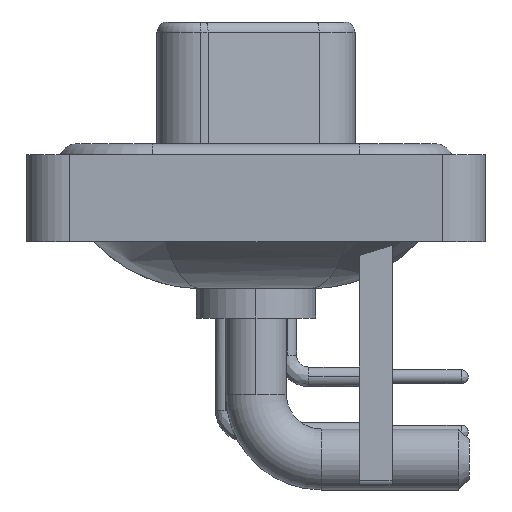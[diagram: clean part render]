
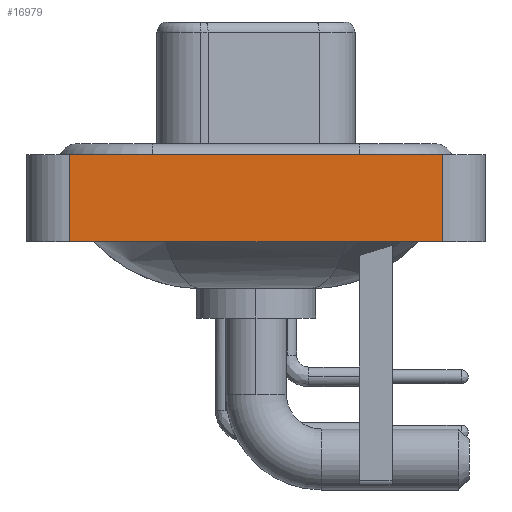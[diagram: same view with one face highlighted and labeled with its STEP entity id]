
A CAD part, left-side view. The second image highlights one B-rep face of the part: STEP entity #16979.
In plain terms, the highlighted planar face has unit normal (-1, 0, 0).
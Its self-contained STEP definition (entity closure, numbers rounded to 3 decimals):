
#830 = PLANE ( 'NONE',  #2655 ) ;
#1372 = LINE ( 'NONE', #16471, #21326 ) ;
#1569 = CARTESIAN_POINT ( 'NONE',  ( -7.3, 8.55, -3.6 ) ) ;
#2655 = AXIS2_PLACEMENT_3D ( 'NONE', #10291, #4549, #4817 ) ;
#2939 = CARTESIAN_POINT ( 'NONE',  ( -7.3, -8.55, 0.4 ) ) ;
#4549 = DIRECTION ( 'NONE',  ( -1., 0., 0. ) ) ;
#4817 = DIRECTION ( 'NONE',  ( 0., 0., 1. ) ) ;
#4832 = ORIENTED_EDGE ( 'NONE', *, *, #13783, .F. ) ;
#4885 = CARTESIAN_POINT ( 'NONE',  ( -7.3, 8.55, -3.6 ) ) ;
#4992 = DIRECTION ( 'NONE',  ( 0., -1., 0. ) ) ;
#5637 = VECTOR ( 'NONE', #4992, 1000. ) ;
#6269 = ORIENTED_EDGE ( 'NONE', *, *, #20563, .T. ) ;
#6390 = VERTEX_POINT ( 'NONE', #25256 ) ;
#6558 = LINE ( 'NONE', #20486, #23531 ) ;
#8976 = DIRECTION ( 'NONE',  ( 0., 0., 1. ) ) ;
#9183 = DIRECTION ( 'NONE',  ( 0., 0., 1. ) ) ;
#9903 = VERTEX_POINT ( 'NONE', #14585 ) ;
#10291 = CARTESIAN_POINT ( 'NONE',  ( -7.3, -8.55, -3.6 ) ) ;
#12181 = DIRECTION ( 'NONE',  ( 0., -1., 0. ) ) ;
#13783 = EDGE_CURVE ( 'NONE', #9903, #20395, #18400, .T. ) ;
#14347 = ORIENTED_EDGE ( 'NONE', *, *, #22357, .F. ) ;
#14585 = CARTESIAN_POINT ( 'NONE',  ( -7.3, 8.55, 0.4 ) ) ;
#14774 = VERTEX_POINT ( 'NONE', #1569 ) ;
#14860 = CARTESIAN_POINT ( 'NONE',  ( -7.3, -8.55, 0.4 ) ) ;
#16471 = CARTESIAN_POINT ( 'NONE',  ( -7.3, -8.55, -3.6 ) ) ;
#16511 = LINE ( 'NONE', #4885, #24943 ) ;
#16979 = ADVANCED_FACE ( 'NONE', ( #24001 ), #830, .T. ) ;
#18400 = LINE ( 'NONE', #2939, #5637 ) ;
#20350 = ORIENTED_EDGE ( 'NONE', *, *, #24303, .T. ) ;
#20395 = VERTEX_POINT ( 'NONE', #14860 ) ;
#20486 = CARTESIAN_POINT ( 'NONE',  ( -7.3, -8.55, -3.6 ) ) ;
#20563 = EDGE_CURVE ( 'NONE', #6390, #20395, #1372, .T. ) ;
#20705 = EDGE_LOOP ( 'NONE', ( #6269, #4832, #14347, #20350 ) ) ;
#21326 = VECTOR ( 'NONE', #9183, 1000. ) ;
#22357 = EDGE_CURVE ( 'NONE', #14774, #9903, #16511, .T. ) ;
#23531 = VECTOR ( 'NONE', #12181, 1000. ) ;
#24001 = FACE_OUTER_BOUND ( 'NONE', #20705, .T. ) ;
#24303 = EDGE_CURVE ( 'NONE', #14774, #6390, #6558, .T. ) ;
#24943 = VECTOR ( 'NONE', #8976, 1000. ) ;
#25256 = CARTESIAN_POINT ( 'NONE',  ( -7.3, -8.55, -3.6 ) ) ;
